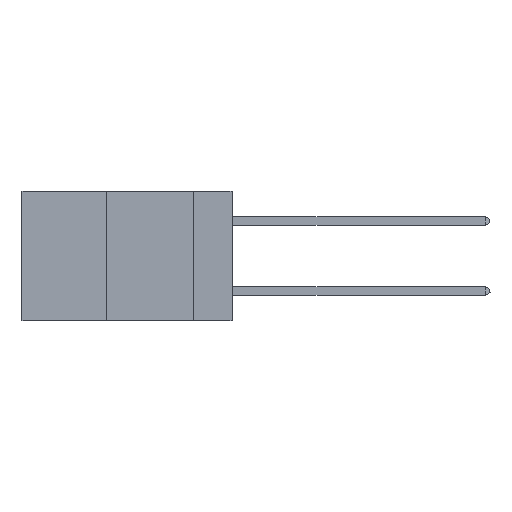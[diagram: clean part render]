
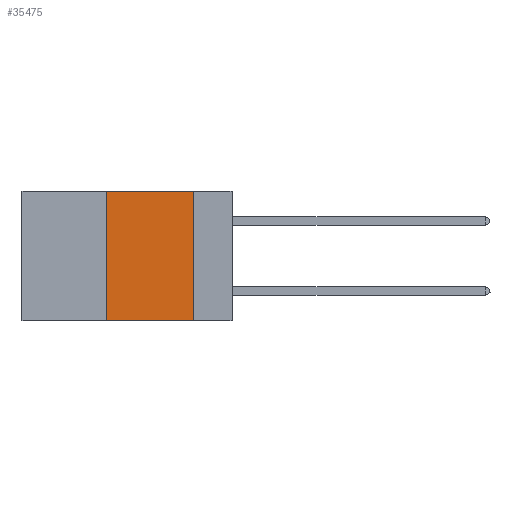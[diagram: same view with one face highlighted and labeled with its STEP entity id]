
A CAD part, left-side view. The second image highlights one B-rep face of the part: STEP entity #35475.
In plain terms, the highlighted planar face has unit normal (-1, 0, 0).
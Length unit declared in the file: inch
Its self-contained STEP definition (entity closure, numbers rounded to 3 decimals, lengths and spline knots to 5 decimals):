
#499 = CARTESIAN_POINT ( 'NONE',  ( 0., 0.6, 0. ) ) ;
#699 = CARTESIAN_POINT ( 'NONE',  ( 0., 0.36, 0. ) ) ;
#3546 = VERTEX_POINT ( 'NONE', #15442 ) ;
#3959 = PLANE ( 'NONE',  #6924 ) ;
#5215 = DIRECTION ( 'NONE',  ( 0., -1., 0. ) ) ;
#5496 = CARTESIAN_POINT ( 'NONE',  ( 0., 0.36, 0. ) ) ;
#6137 = CARTESIAN_POINT ( 'NONE',  ( 0., 0.6, 0. ) ) ;
#6530 = EDGE_CURVE ( 'NONE', #24953, #3546, #41091, .T. ) ;
#6924 = AXIS2_PLACEMENT_3D ( 'NONE', #499, #41843, #31732 ) ;
#10188 = DIRECTION ( 'NONE',  ( 0., 0., -1. ) ) ;
#10828 = LINE ( 'NONE', #6137, #40677 ) ;
#13338 = EDGE_LOOP ( 'NONE', ( #40114, #43243, #29608, #14469 ) ) ;
#13448 = VECTOR ( 'NONE', #5215, 39.37008 ) ;
#14469 = ORIENTED_EDGE ( 'NONE', *, *, #6530, .T. ) ;
#14652 = DIRECTION ( 'NONE',  ( 0., 0., 1. ) ) ;
#15241 = FACE_OUTER_BOUND ( 'NONE', #13338, .T. ) ;
#15442 = CARTESIAN_POINT ( 'NONE',  ( 0., 0.11, -0.37 ) ) ;
#17082 = VERTEX_POINT ( 'NONE', #36139 ) ;
#24953 = VERTEX_POINT ( 'NONE', #25180 ) ;
#25052 = VECTOR ( 'NONE', #14652, 39.37008 ) ;
#25180 = CARTESIAN_POINT ( 'NONE',  ( 0., 0.36, -0.37 ) ) ;
#26750 = DIRECTION ( 'NONE',  ( 0., -1., 0. ) ) ;
#29608 = ORIENTED_EDGE ( 'NONE', *, *, #44317, .F. ) ;
#31732 = DIRECTION ( 'NONE',  ( 0., 0., -1. ) ) ;
#34154 = CARTESIAN_POINT ( 'NONE',  ( 0., 0.11, 0. ) ) ;
#34228 = VECTOR ( 'NONE', #10188, 39.37008 ) ;
#35366 = EDGE_CURVE ( 'NONE', #17082, #3546, #43420, .T. ) ;
#35475 = ADVANCED_FACE ( 'NONE', ( #15241 ), #3959, .F. ) ;
#36139 = CARTESIAN_POINT ( 'NONE',  ( 0., 0.11, 0. ) ) ;
#37417 = EDGE_CURVE ( 'NONE', #40763, #17082, #10828, .T. ) ;
#40114 = ORIENTED_EDGE ( 'NONE', *, *, #35366, .F. ) ;
#40677 = VECTOR ( 'NONE', #26750, 39.37008 ) ;
#40763 = VERTEX_POINT ( 'NONE', #5496 ) ;
#41091 = LINE ( 'NONE', #42978, #13448 ) ;
#41843 = DIRECTION ( 'NONE',  ( 1., 0., 0. ) ) ;
#42887 = LINE ( 'NONE', #699, #25052 ) ;
#42978 = CARTESIAN_POINT ( 'NONE',  ( 0., 0.6, -0.37 ) ) ;
#43243 = ORIENTED_EDGE ( 'NONE', *, *, #37417, .F. ) ;
#43420 = LINE ( 'NONE', #34154, #34228 ) ;
#44317 = EDGE_CURVE ( 'NONE', #24953, #40763, #42887, .T. ) ;
